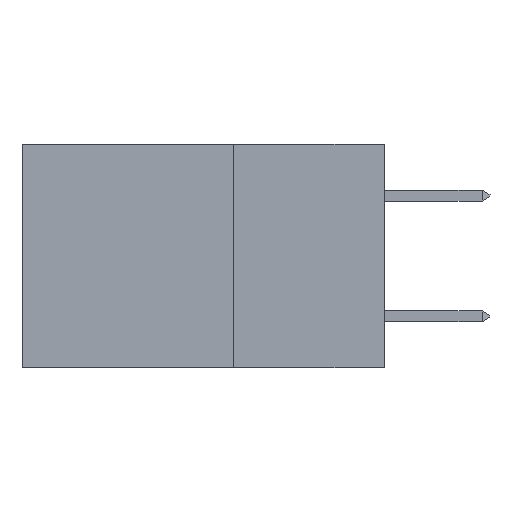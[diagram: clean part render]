
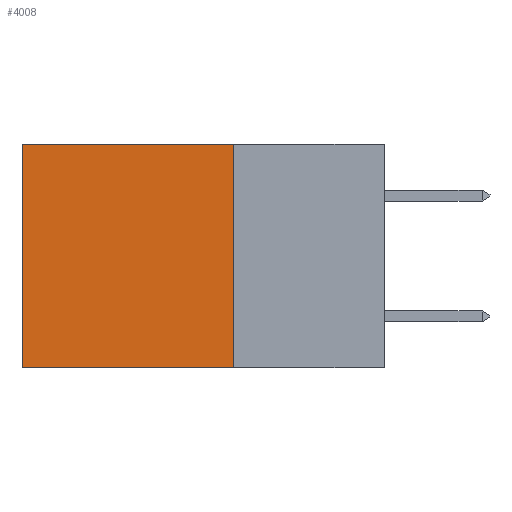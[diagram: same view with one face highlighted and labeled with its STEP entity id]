
A CAD part, left-side view. The second image highlights one B-rep face of the part: STEP entity #4008.
In plain terms, the highlighted planar face has unit normal (-1, 0, 0).
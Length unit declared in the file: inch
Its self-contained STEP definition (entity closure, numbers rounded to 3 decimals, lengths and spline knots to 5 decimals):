
#114 = VERTEX_POINT ( 'NONE', #519 ) ;
#519 = CARTESIAN_POINT ( 'NONE',  ( 0.2875, 0.25, -0.37 ) ) ;
#549 = ORIENTED_EDGE ( 'NONE', *, *, #15578, .F. ) ;
#984 = ORIENTED_EDGE ( 'NONE', *, *, #12627, .T. ) ;
#1566 = VECTOR ( 'NONE', #4988, 39.37008 ) ;
#2060 = DIRECTION ( 'NONE',  ( 0., 1., 0. ) ) ;
#3193 = VECTOR ( 'NONE', #5129, 39.37008 ) ;
#3913 = VECTOR ( 'NONE', #2060, 39.37008 ) ;
#4008 = ADVANCED_FACE ( 'NONE', ( #9273 ), #9985, .F. ) ;
#4988 = DIRECTION ( 'NONE',  ( 0., 1., 0. ) ) ;
#5129 = DIRECTION ( 'NONE',  ( 0., 0., -1. ) ) ;
#5192 = VERTEX_POINT ( 'NONE', #15799 ) ;
#6072 = ORIENTED_EDGE ( 'NONE', *, *, #11431, .T. ) ;
#6933 = VERTEX_POINT ( 'NONE', #14069 ) ;
#6995 = CARTESIAN_POINT ( 'NONE',  ( 0.2875, 0.25, 0. ) ) ;
#7312 = VERTEX_POINT ( 'NONE', #12304 ) ;
#9273 = FACE_OUTER_BOUND ( 'NONE', #14738, .T. ) ;
#9431 = AXIS2_PLACEMENT_3D ( 'NONE', #6995, #12667, #15599 ) ;
#9985 = PLANE ( 'NONE',  #9431 ) ;
#10692 = EDGE_CURVE ( 'NONE', #7312, #114, #15205, .T. ) ;
#11063 = DIRECTION ( 'NONE',  ( 0., 0., -1. ) ) ;
#11294 = VECTOR ( 'NONE', #11063, 39.37008 ) ;
#11313 = ORIENTED_EDGE ( 'NONE', *, *, #10692, .F. ) ;
#11431 = EDGE_CURVE ( 'NONE', #7312, #5192, #17178, .T. ) ;
#12121 = CARTESIAN_POINT ( 'NONE',  ( 0.2875, 0.25, 0. ) ) ;
#12304 = CARTESIAN_POINT ( 'NONE',  ( 0.2875, 0.25, 0. ) ) ;
#12627 = EDGE_CURVE ( 'NONE', #5192, #6933, #15565, .T. ) ;
#12667 = DIRECTION ( 'NONE',  ( 1., 0., 0. ) ) ;
#14069 = CARTESIAN_POINT ( 'NONE',  ( 0.2875, 0.6, -0.37 ) ) ;
#14583 = LINE ( 'NONE', #17608, #3913 ) ;
#14738 = EDGE_LOOP ( 'NONE', ( #984, #549, #11313, #6072 ) ) ;
#15205 = LINE ( 'NONE', #16729, #3193 ) ;
#15565 = LINE ( 'NONE', #18330, #11294 ) ;
#15578 = EDGE_CURVE ( 'NONE', #114, #6933, #14583, .T. ) ;
#15599 = DIRECTION ( 'NONE',  ( 0., 0., -1. ) ) ;
#15799 = CARTESIAN_POINT ( 'NONE',  ( 0.2875, 0.6, 0. ) ) ;
#16729 = CARTESIAN_POINT ( 'NONE',  ( 0.2875, 0.25, 0. ) ) ;
#17178 = LINE ( 'NONE', #12121, #1566 ) ;
#17608 = CARTESIAN_POINT ( 'NONE',  ( 0.2875, 0.25, -0.37 ) ) ;
#18330 = CARTESIAN_POINT ( 'NONE',  ( 0.2875, 0.6, 0. ) ) ;
